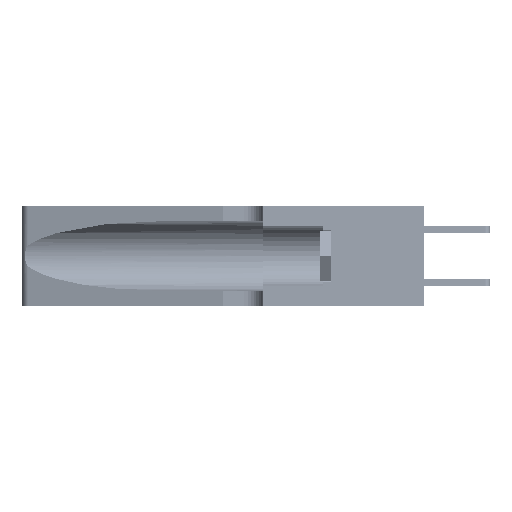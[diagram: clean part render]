
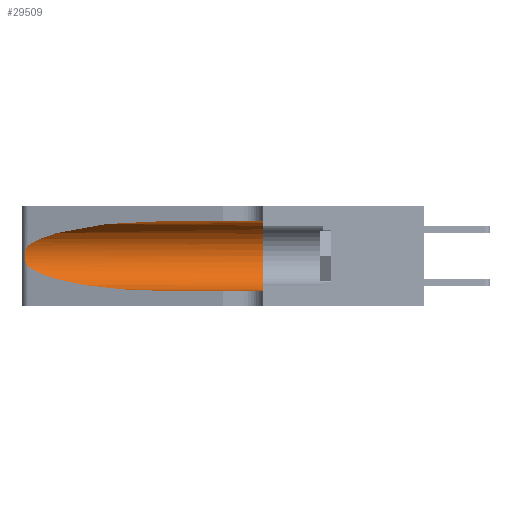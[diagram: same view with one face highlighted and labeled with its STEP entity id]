
A CAD part, left-side view. The second image highlights one B-rep face of the part: STEP entity #29509.
In plain terms, the highlighted cylindrical face has radius 3.308 mm (diameter 6.617 mm), a partial arc.
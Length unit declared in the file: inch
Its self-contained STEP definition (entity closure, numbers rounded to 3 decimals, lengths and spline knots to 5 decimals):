
#459 = VERTEX_POINT ( 'NONE', #6870 ) ;
#2333 = EDGE_CURVE ( 'NONE', #40396, #11056, #15143, .T. ) ;
#3464 = ORIENTED_EDGE ( 'NONE', *, *, #2333, .T. ) ;
#3533 = CARTESIAN_POINT ( 'NONE',  ( 0.26075, 1.23896, 0.19203 ) ) ;
#4028 = ORIENTED_EDGE ( 'NONE', *, *, #32063, .T. ) ;
#4230 = VERTEX_POINT ( 'NONE', #23196 ) ;
#5306 = LINE ( 'NONE', #34227, #7143 ) ;
#6535 = DIRECTION ( 'NONE',  ( 0., -1., 0. ) ) ;
#6870 = CARTESIAN_POINT ( 'NONE',  ( 0.1305, 0.72297, 0.05475 ) ) ;
#7143 = VECTOR ( 'NONE', #14702, 39.37008 ) ;
#7661 = CARTESIAN_POINT ( 'NONE',  ( 0.25487, 1.22718, 0.22369 ) ) ;
#11056 = VERTEX_POINT ( 'NONE', #7661 ) ;
#11613 = CARTESIAN_POINT ( 'NONE',  ( 0.25487, 1.22718, 0.22369 ) ) ;
#11743 = CARTESIAN_POINT ( 'NONE',  ( 0.26018, 1.23835, 0.19895 ) ) ;
#12054 = LINE ( 'NONE', #30672, #16957 ) ;
#12993 = CIRCLE ( 'NONE', #29424, 0.13025 ) ;
#14019 = CARTESIAN_POINT ( 'NONE',  ( 0.18966, 0.96281, 0.31525 ) ) ;
#14572 = CARTESIAN_POINT ( 'NONE',  ( 0.1305, 1.61858, 0.185 ) ) ;
#14702 = DIRECTION ( 'NONE',  ( 0., -1., 0. ) ) ;
#15143 =( BOUNDED_CURVE ( )  B_SPLINE_CURVE ( 3, ( #18459, #14019, #25846, #11613 ),
 .UNSPECIFIED., .F., .F. ) 
 B_SPLINE_CURVE_WITH_KNOTS ( ( 4, 4 ),
 ( 1.5708, 2.84003 ),
 .UNSPECIFIED. ) 
 CURVE ( )  GEOMETRIC_REPRESENTATION_ITEM ( )  RATIONAL_B_SPLINE_CURVE ( ( 1., 0.87, 0.87, 1. ) ) 
 REPRESENTATION_ITEM ( '' )  );
#15154 = CARTESIAN_POINT ( 'NONE',  ( 0.25487, 1.22718, 0.14631 ) ) ;
#16731 = CARTESIAN_POINT ( 'NONE',  ( 0.1305, 0.35, 0.185 ) ) ;
#16837 = EDGE_CURVE ( 'NONE', #33435, #46550, #12993, .T. ) ;
#16957 = VECTOR ( 'NONE', #23126, 39.37008 ) ;
#18459 = CARTESIAN_POINT ( 'NONE',  ( 0.1305, 0.72297, 0.31525 ) ) ;
#19499 = ORIENTED_EDGE ( 'NONE', *, *, #16837, .F. ) ;
#19664 = CARTESIAN_POINT ( 'NONE',  ( 0.25856, 1.23593, 0.16098 ) ) ;
#20408 = EDGE_CURVE ( 'NONE', #4230, #459, #37770, .T. ) ;
#20662 = DIRECTION ( 'NONE',  ( 0., 0., 1. ) ) ;
#22591 = ORIENTED_EDGE ( 'NONE', *, *, #32605, .F. ) ;
#23019 = CARTESIAN_POINT ( 'NONE',  ( 0.25789, 1.23486, 0.15765 ) ) ;
#23093 = DIRECTION ( 'NONE',  ( 0., 0., -1. ) ) ;
#23126 = DIRECTION ( 'NONE',  ( 0., -1., 0. ) ) ;
#23196 = CARTESIAN_POINT ( 'NONE',  ( 0.25487, 1.22718, 0.14631 ) ) ;
#23709 = CARTESIAN_POINT ( 'NONE',  ( 0.25854, 1.2359, 0.20912 ) ) ;
#25846 = CARTESIAN_POINT ( 'NONE',  ( 0.2373, 1.15595, 0.28018 ) ) ;
#25911 = EDGE_CURVE ( 'NONE', #11056, #4230, #38700, .T. ) ;
#26477 = CARTESIAN_POINT ( 'NONE',  ( 0.25555, 1.22994, 0.2215 ) ) ;
#27627 = CARTESIAN_POINT ( 'NONE',  ( 0.25639, 1.23186, 0.15144 ) ) ;
#29424 = AXIS2_PLACEMENT_3D ( 'NONE', #16731, #40730, #20662 ) ;
#29509 = ADVANCED_FACE ( 'NONE', ( #39476 ), #44964, .F. ) ;
#29751 = CARTESIAN_POINT ( 'NONE',  ( 0.1305, 0.72297, 0.31525 ) ) ;
#30672 = CARTESIAN_POINT ( 'NONE',  ( 0.1305, 1.61858, 0.05475 ) ) ;
#31245 = CARTESIAN_POINT ( 'NONE',  ( 0.25555, 1.22993, 0.14849 ) ) ;
#31735 = AXIS2_PLACEMENT_3D ( 'NONE', #14572, #6535, #23093 ) ;
#32063 = EDGE_CURVE ( 'NONE', #459, #46550, #12054, .T. ) ;
#32605 = EDGE_CURVE ( 'NONE', #40396, #33435, #5306, .T. ) ;
#33435 = VERTEX_POINT ( 'NONE', #40300 ) ;
#34227 = CARTESIAN_POINT ( 'NONE',  ( 0.1305, 1.61858, 0.31525 ) ) ;
#34684 = CARTESIAN_POINT ( 'NONE',  ( 0.26075, 1.23896, 0.178 ) ) ;
#34857 = CARTESIAN_POINT ( 'NONE',  ( 0.25787, 1.23484, 0.2124 ) ) ;
#37770 =( BOUNDED_CURVE ( )  B_SPLINE_CURVE ( 3, ( #44749, #45071, #48656, #45240 ),
 .UNSPECIFIED., .F., .F. ) 
 B_SPLINE_CURVE_WITH_KNOTS ( ( 4, 4 ),
 ( 3.44316, 4.71239 ),
 .UNSPECIFIED. ) 
 CURVE ( )  GEOMETRIC_REPRESENTATION_ITEM ( )  RATIONAL_B_SPLINE_CURVE ( ( 1., 0.87, 0.87, 1. ) ) 
 REPRESENTATION_ITEM ( '' )  );
#38700 = B_SPLINE_CURVE_WITH_KNOTS ( 'NONE', 3,
 ( #42073, #26477, #39162, #34857, #23709, #11743, #3533, #34684, #42749, #19664, #23019, #27627, #31245, #15154 ),
 .UNSPECIFIED., .F., .F.,
 ( 4, 2, 2, 2, 2, 2, 4 ),
 ( 0., 0.00027, 0.00053, 0.00107, 0.0016, 0.00187, 0.00214 ),
 .UNSPECIFIED. ) ;
#39162 = CARTESIAN_POINT ( 'NONE',  ( 0.25639, 1.23184, 0.21858 ) ) ;
#39476 = FACE_OUTER_BOUND ( 'NONE', #48251, .T. ) ;
#40045 = CARTESIAN_POINT ( 'NONE',  ( 0.1305, 0.35, 0.05475 ) ) ;
#40300 = CARTESIAN_POINT ( 'NONE',  ( 0.1305, 0.35, 0.31525 ) ) ;
#40396 = VERTEX_POINT ( 'NONE', #29751 ) ;
#40730 = DIRECTION ( 'NONE',  ( 0., 1., 0. ) ) ;
#41043 = ORIENTED_EDGE ( 'NONE', *, *, #25911, .T. ) ;
#42073 = CARTESIAN_POINT ( 'NONE',  ( 0.25487, 1.22718, 0.22369 ) ) ;
#42749 = CARTESIAN_POINT ( 'NONE',  ( 0.26017, 1.23833, 0.17102 ) ) ;
#44749 = CARTESIAN_POINT ( 'NONE',  ( 0.25487, 1.22718, 0.14631 ) ) ;
#44964 = CYLINDRICAL_SURFACE ( 'NONE', #31735, 0.13025 ) ;
#45071 = CARTESIAN_POINT ( 'NONE',  ( 0.2373, 1.15595, 0.08982 ) ) ;
#45240 = CARTESIAN_POINT ( 'NONE',  ( 0.1305, 0.72297, 0.05475 ) ) ;
#46550 = VERTEX_POINT ( 'NONE', #40045 ) ;
#48251 = EDGE_LOOP ( 'NONE', ( #3464, #41043, #50183, #4028, #19499, #22591 ) ) ;
#48656 = CARTESIAN_POINT ( 'NONE',  ( 0.18966, 0.96281, 0.05475 ) ) ;
#50183 = ORIENTED_EDGE ( 'NONE', *, *, #20408, .T. ) ;
